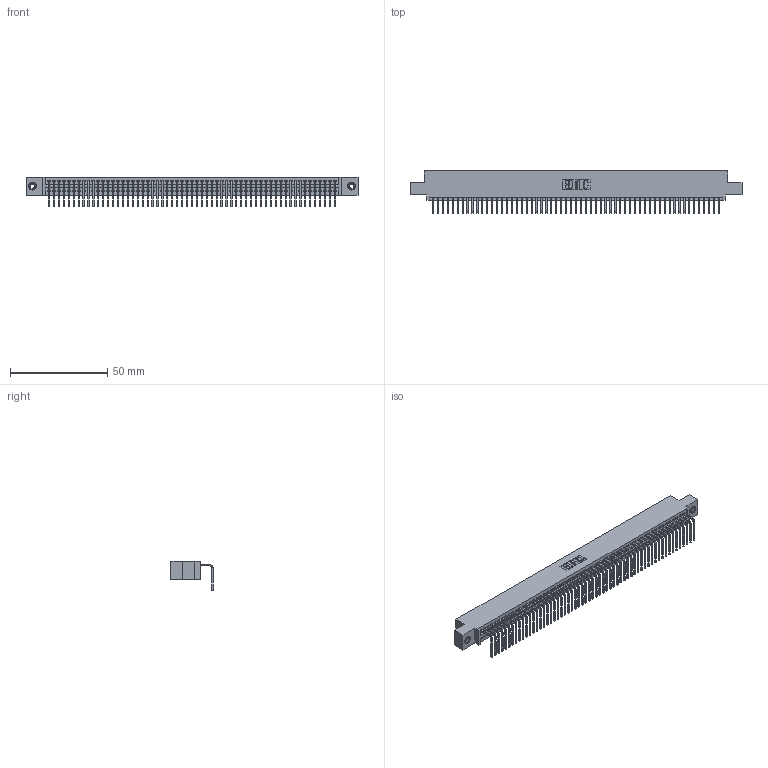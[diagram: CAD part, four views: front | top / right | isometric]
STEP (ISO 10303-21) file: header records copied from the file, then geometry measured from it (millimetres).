
FILE_DESCRIPTION (( 'STEP AP203' ), '1' );
FILE_NAME ('395-059-558-408.STEP', '2018-11-23T09:46:41', ( '' ), ( '' ), 'SwSTEP 2.0', 'SolidWorks 2016', '' );
FILE_SCHEMA (( 'CONFIG_CONTROL_DESIGN' ));
Length unit declared in the file: inch
Products named in the file (4): 345 Part_0.110 Offset - 0.156 Dia-TI; 395-059-558-408; 345-292-001_558 Tail - 2; 345-250-001_345-250-003-102
Assembly tree (62 placements, depth 2):
  395-059-558-408
    345 Part_0.110 Offset - 0.156 Dia-TI
    345-292-001_558 Tail - 2  x59
    345-250-001_345-250-003-102  x2
Bounding box: 171.07 x 21.83 x 15.37 mm (x, y, z)
Volume: 16504.3 mm3; surface area: 23419.8 mm2
Topology: 62 solids, 62 shells, 3730 faces, 11227 edges, 7398 vertices
Faces by surface type: plane 2594, cylinder 1120, cone 12, torus 4
Entity records: 43518 total; most frequent: CARTESIAN_POINT 7520, ORIENTED_EDGE 7506, DIRECTION 6569, EDGE_CURVE 3753, VECTOR 3365, LINE 3365, VERTEX_POINT 2496, AXIS2_PLACEMENT_3D 1602
